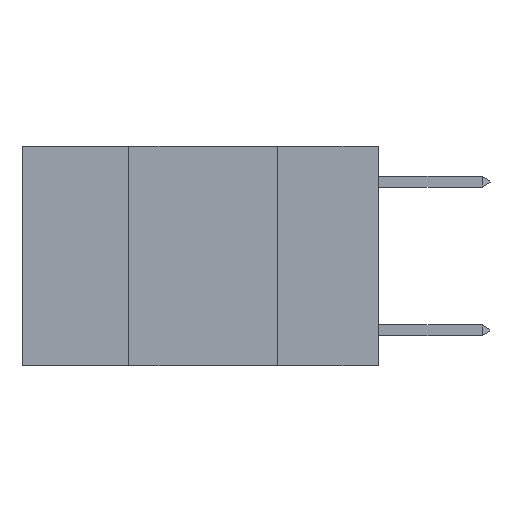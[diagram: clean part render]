
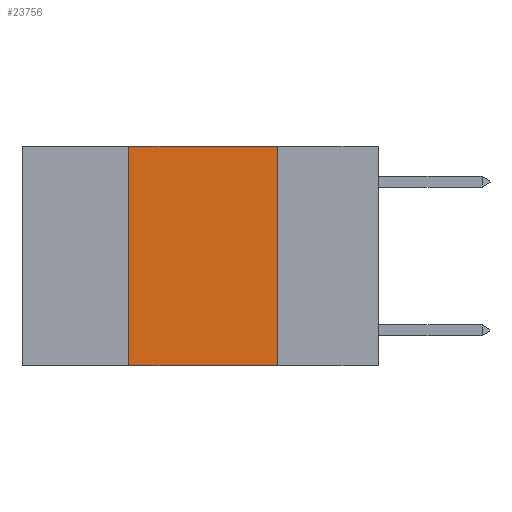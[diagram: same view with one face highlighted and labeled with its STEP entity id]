
A CAD part, left-side view. The second image highlights one B-rep face of the part: STEP entity #23756.
In plain terms, the highlighted planar face has unit normal (-1, 0, 0).
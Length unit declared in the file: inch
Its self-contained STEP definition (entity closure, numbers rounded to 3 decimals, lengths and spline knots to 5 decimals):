
#492 = VERTEX_POINT ( 'NONE', #3208 ) ;
#3208 = CARTESIAN_POINT ( 'NONE',  ( 0., 0.17, 0. ) ) ;
#3213 = CARTESIAN_POINT ( 'NONE',  ( 0., 0.17, -0.37 ) ) ;
#3539 = ORIENTED_EDGE ( 'NONE', *, *, #27156, .F. ) ;
#4227 = AXIS2_PLACEMENT_3D ( 'NONE', #10153, #12249, #26955 ) ;
#4368 = FACE_OUTER_BOUND ( 'NONE', #21784, .T. ) ;
#4531 = VECTOR ( 'NONE', #13807, 39.37008 ) ;
#5058 = DIRECTION ( 'NONE',  ( 0., 0., -1. ) ) ;
#6731 = DIRECTION ( 'NONE',  ( 0., -1., 0. ) ) ;
#8078 = PLANE ( 'NONE',  #4227 ) ;
#8668 = VECTOR ( 'NONE', #6731, 39.37008 ) ;
#8734 = CARTESIAN_POINT ( 'NONE',  ( 0., 0.6, 0. ) ) ;
#8975 = VERTEX_POINT ( 'NONE', #25183 ) ;
#9130 = ORIENTED_EDGE ( 'NONE', *, *, #13411, .T. ) ;
#9265 = VERTEX_POINT ( 'NONE', #26160 ) ;
#9308 = LINE ( 'NONE', #8734, #8668 ) ;
#10153 = CARTESIAN_POINT ( 'NONE',  ( 0., 0.6, 0. ) ) ;
#12153 = LINE ( 'NONE', #23882, #16397 ) ;
#12184 = VECTOR ( 'NONE', #22592, 39.37008 ) ;
#12249 = DIRECTION ( 'NONE',  ( 1., 0., 0. ) ) ;
#12700 = ORIENTED_EDGE ( 'NONE', *, *, #13935, .F. ) ;
#13411 = EDGE_CURVE ( 'NONE', #9265, #20187, #17747, .T. ) ;
#13719 = CARTESIAN_POINT ( 'NONE',  ( 0., 0.42, 0. ) ) ;
#13807 = DIRECTION ( 'NONE',  ( 0., 0., 1. ) ) ;
#13935 = EDGE_CURVE ( 'NONE', #492, #20187, #12153, .T. ) ;
#15637 = LINE ( 'NONE', #13719, #4531 ) ;
#16397 = VECTOR ( 'NONE', #5058, 39.37008 ) ;
#17747 = LINE ( 'NONE', #26689, #12184 ) ;
#20187 = VERTEX_POINT ( 'NONE', #3213 ) ;
#21784 = EDGE_LOOP ( 'NONE', ( #12700, #24577, #3539, #9130 ) ) ;
#22592 = DIRECTION ( 'NONE',  ( 0., -1., 0. ) ) ;
#23319 = EDGE_CURVE ( 'NONE', #8975, #492, #9308, .T. ) ;
#23756 = ADVANCED_FACE ( 'NONE', ( #4368 ), #8078, .F. ) ;
#23882 = CARTESIAN_POINT ( 'NONE',  ( 0., 0.17, 0. ) ) ;
#24577 = ORIENTED_EDGE ( 'NONE', *, *, #23319, .F. ) ;
#25183 = CARTESIAN_POINT ( 'NONE',  ( 0., 0.42, 0. ) ) ;
#26160 = CARTESIAN_POINT ( 'NONE',  ( 0., 0.42, -0.37 ) ) ;
#26689 = CARTESIAN_POINT ( 'NONE',  ( 0., 0.6, -0.37 ) ) ;
#26955 = DIRECTION ( 'NONE',  ( 0., 0., -1. ) ) ;
#27156 = EDGE_CURVE ( 'NONE', #9265, #8975, #15637, .T. ) ;
